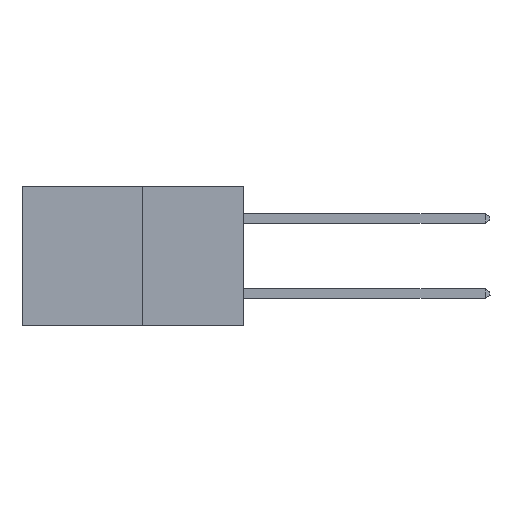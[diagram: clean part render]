
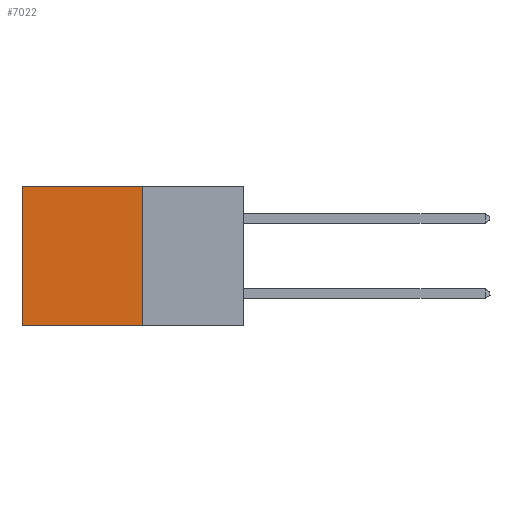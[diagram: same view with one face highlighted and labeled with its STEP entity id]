
A CAD part, left-side view. The second image highlights one B-rep face of the part: STEP entity #7022.
In plain terms, the highlighted planar face has unit normal (-1, 0, 0).
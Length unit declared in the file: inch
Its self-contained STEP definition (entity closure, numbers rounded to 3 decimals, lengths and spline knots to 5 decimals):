
#301 = LINE ( 'NONE', #15632, #16318 ) ;
#749 = CARTESIAN_POINT ( 'NONE',  ( 0.277, 0.27, -0.37 ) ) ;
#2545 = VECTOR ( 'NONE', #25176, 39.37008 ) ;
#4100 = VERTEX_POINT ( 'NONE', #749 ) ;
#5002 = PLANE ( 'NONE',  #6490 ) ;
#5125 = DIRECTION ( 'NONE',  ( 0., 0., -1. ) ) ;
#5466 = EDGE_CURVE ( 'NONE', #11937, #22869, #20369, .T. ) ;
#6490 = AXIS2_PLACEMENT_3D ( 'NONE', #21672, #15421, #9168 ) ;
#7022 = ADVANCED_FACE ( 'NONE', ( #8098 ), #5002, .F. ) ;
#7488 = EDGE_CURVE ( 'NONE', #11937, #4100, #19240, .T. ) ;
#7992 = ORIENTED_EDGE ( 'NONE', *, *, #13568, .F. ) ;
#8098 = FACE_OUTER_BOUND ( 'NONE', #11783, .T. ) ;
#9168 = DIRECTION ( 'NONE',  ( 0., 0., -1. ) ) ;
#10703 = ORIENTED_EDGE ( 'NONE', *, *, #5466, .T. ) ;
#10813 = ORIENTED_EDGE ( 'NONE', *, *, #23800, .T. ) ;
#11783 = EDGE_LOOP ( 'NONE', ( #10813, #7992, #17133, #10703 ) ) ;
#11937 = VERTEX_POINT ( 'NONE', #15138 ) ;
#13037 = CARTESIAN_POINT ( 'NONE',  ( 0.277, 0.27, -0.37 ) ) ;
#13568 = EDGE_CURVE ( 'NONE', #4100, #17909, #19916, .T. ) ;
#15138 = CARTESIAN_POINT ( 'NONE',  ( 0.277, 0.27, 0. ) ) ;
#15421 = DIRECTION ( 'NONE',  ( 1., 0., 0. ) ) ;
#15632 = CARTESIAN_POINT ( 'NONE',  ( 0.277, 0.59, -0.37 ) ) ;
#16318 = VECTOR ( 'NONE', #5125, 39.37008 ) ;
#16458 = DIRECTION ( 'NONE',  ( 0., 1., 0. ) ) ;
#17057 = CARTESIAN_POINT ( 'NONE',  ( 0.277, 0.27, 0. ) ) ;
#17133 = ORIENTED_EDGE ( 'NONE', *, *, #7488, .F. ) ;
#17240 = DIRECTION ( 'NONE',  ( 0., 1., 0. ) ) ;
#17909 = VERTEX_POINT ( 'NONE', #21659 ) ;
#18874 = CARTESIAN_POINT ( 'NONE',  ( 0.277, 0.27, -0.37 ) ) ;
#19030 = VECTOR ( 'NONE', #16458, 39.37008 ) ;
#19240 = LINE ( 'NONE', #18874, #2545 ) ;
#19916 = LINE ( 'NONE', #13037, #24783 ) ;
#20369 = LINE ( 'NONE', #17057, #19030 ) ;
#21293 = CARTESIAN_POINT ( 'NONE',  ( 0.277, 0.59, 0. ) ) ;
#21659 = CARTESIAN_POINT ( 'NONE',  ( 0.277, 0.59, -0.37 ) ) ;
#21672 = CARTESIAN_POINT ( 'NONE',  ( 0.277, 0.27, -0.37 ) ) ;
#22869 = VERTEX_POINT ( 'NONE', #21293 ) ;
#23800 = EDGE_CURVE ( 'NONE', #22869, #17909, #301, .T. ) ;
#24783 = VECTOR ( 'NONE', #17240, 39.37008 ) ;
#25176 = DIRECTION ( 'NONE',  ( 0., 0., -1. ) ) ;
